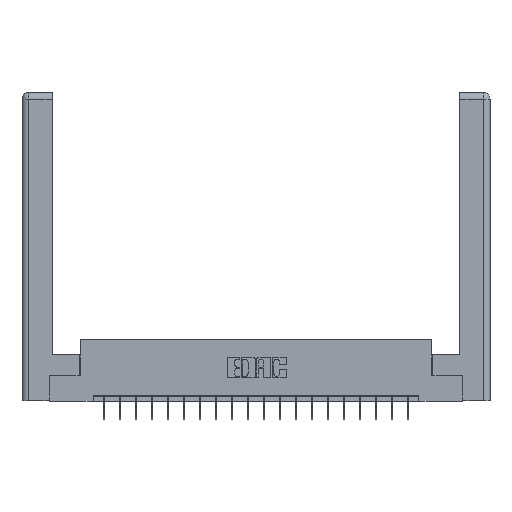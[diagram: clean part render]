
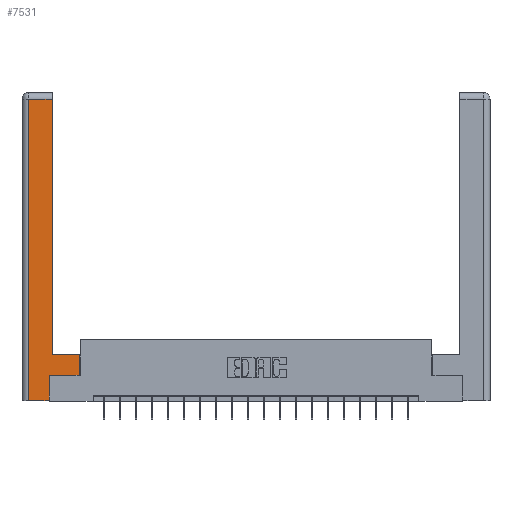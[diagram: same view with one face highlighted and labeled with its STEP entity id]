
A CAD part, top view. The second image highlights one B-rep face of the part: STEP entity #7531.
In plain terms, the highlighted planar face has unit normal (0, 0, 1).
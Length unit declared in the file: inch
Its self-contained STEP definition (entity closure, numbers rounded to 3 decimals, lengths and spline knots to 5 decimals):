
#225 = CARTESIAN_POINT ( 'NONE',  ( 0.265, 0.245, 0. ) ) ;
#317 = CARTESIAN_POINT ( 'NONE',  ( 0.0615, 0., 0. ) ) ;
#633 = DIRECTION ( 'NONE',  ( 1., 0., 0. ) ) ;
#900 = ORIENTED_EDGE ( 'NONE', *, *, #13236, .T. ) ;
#982 = CARTESIAN_POINT ( 'NONE',  ( 0.0615, 0., 0. ) ) ;
#1739 = VECTOR ( 'NONE', #633, 39.37008 ) ;
#1836 = VERTEX_POINT ( 'NONE', #8463 ) ;
#1854 = EDGE_CURVE ( 'NONE', #6002, #17932, #10151, .T. ) ;
#2524 = LINE ( 'NONE', #225, #17028 ) ;
#2531 = CARTESIAN_POINT ( 'NONE',  ( 0.0615, 2.94, 0. ) ) ;
#2778 = ORIENTED_EDGE ( 'NONE', *, *, #16266, .T. ) ;
#3439 = DIRECTION ( 'NONE',  ( 0., 0., -1. ) ) ;
#3519 = VERTEX_POINT ( 'NONE', #13654 ) ;
#3767 = CARTESIAN_POINT ( 'NONE',  ( 0.565, 0.45, 0. ) ) ;
#4159 = DIRECTION ( 'NONE',  ( -1., 0., 0. ) ) ;
#4185 = DIRECTION ( 'NONE',  ( 0., -1., 0. ) ) ;
#5205 = CARTESIAN_POINT ( 'NONE',  ( 0., 0., 0. ) ) ;
#5791 = CARTESIAN_POINT ( 'NONE',  ( 0.0615, 2.94, 0. ) ) ;
#5949 = ORIENTED_EDGE ( 'NONE', *, *, #10541, .T. ) ;
#5978 = AXIS2_PLACEMENT_3D ( 'NONE', #5205, #3439, #8343 ) ;
#6002 = VERTEX_POINT ( 'NONE', #16524 ) ;
#6455 = LINE ( 'NONE', #2531, #10020 ) ;
#7178 = VERTEX_POINT ( 'NONE', #7567 ) ;
#7236 = LINE ( 'NONE', #982, #13884 ) ;
#7531 = ADVANCED_FACE ( 'NONE', ( #19474 ), #18111, .F. ) ;
#7567 = CARTESIAN_POINT ( 'NONE',  ( 0.295, 2.94, 0. ) ) ;
#8107 = VERTEX_POINT ( 'NONE', #18086 ) ;
#8117 = LINE ( 'NONE', #13614, #1739 ) ;
#8343 = DIRECTION ( 'NONE',  ( -1., 0., 0. ) ) ;
#8373 = EDGE_LOOP ( 'NONE', ( #9507, #20205, #2778, #11912, #5949, #18914, #19604, #900 ) ) ;
#8411 = EDGE_CURVE ( 'NONE', #3519, #7178, #18422, .T. ) ;
#8463 = CARTESIAN_POINT ( 'NONE',  ( 0.265, 0.245, 0. ) ) ;
#8599 = CARTESIAN_POINT ( 'NONE',  ( 0.565, 0.45, 0. ) ) ;
#8881 = VECTOR ( 'NONE', #12105, 39.37008 ) ;
#9274 = LINE ( 'NONE', #15005, #18453 ) ;
#9507 = ORIENTED_EDGE ( 'NONE', *, *, #8411, .T. ) ;
#9956 = VERTEX_POINT ( 'NONE', #317 ) ;
#10020 = VECTOR ( 'NONE', #4159, 39.37008 ) ;
#10151 = LINE ( 'NONE', #3767, #8881 ) ;
#10386 = DIRECTION ( 'NONE',  ( 0., 1., 0. ) ) ;
#10541 = EDGE_CURVE ( 'NONE', #8107, #1836, #2524, .T. ) ;
#11912 = ORIENTED_EDGE ( 'NONE', *, *, #16694, .T. ) ;
#11979 = DIRECTION ( 'NONE',  ( -1., 0., 0. ) ) ;
#12105 = DIRECTION ( 'NONE',  ( 0., 1., 0. ) ) ;
#12991 = DIRECTION ( 'NONE',  ( 0., 1., 0. ) ) ;
#13236 = EDGE_CURVE ( 'NONE', #17932, #3519, #13496, .T. ) ;
#13265 = EDGE_CURVE ( 'NONE', #1836, #6002, #8117, .T. ) ;
#13496 = LINE ( 'NONE', #18169, #18574 ) ;
#13614 = CARTESIAN_POINT ( 'NONE',  ( 0.565, 0.245, 0. ) ) ;
#13654 = CARTESIAN_POINT ( 'NONE',  ( 0.295, 0.45, 0. ) ) ;
#13838 = VECTOR ( 'NONE', #10386, 39.37008 ) ;
#13884 = VECTOR ( 'NONE', #4185, 39.37008 ) ;
#15005 = CARTESIAN_POINT ( 'NONE',  ( 0.265, 0., 0. ) ) ;
#15440 = CARTESIAN_POINT ( 'NONE',  ( 0.295, 3., 0. ) ) ;
#16266 = EDGE_CURVE ( 'NONE', #16832, #9956, #7236, .T. ) ;
#16524 = CARTESIAN_POINT ( 'NONE',  ( 0.565, 0.245, 0. ) ) ;
#16619 = DIRECTION ( 'NONE',  ( 1., 0., 0. ) ) ;
#16694 = EDGE_CURVE ( 'NONE', #9956, #8107, #9274, .T. ) ;
#16813 = EDGE_CURVE ( 'NONE', #7178, #16832, #6455, .T. ) ;
#16832 = VERTEX_POINT ( 'NONE', #5791 ) ;
#17028 = VECTOR ( 'NONE', #12991, 39.37008 ) ;
#17932 = VERTEX_POINT ( 'NONE', #8599 ) ;
#18086 = CARTESIAN_POINT ( 'NONE',  ( 0.265, 0., 0. ) ) ;
#18111 = PLANE ( 'NONE',  #5978 ) ;
#18169 = CARTESIAN_POINT ( 'NONE',  ( 0.295, 0.45, 0. ) ) ;
#18422 = LINE ( 'NONE', #15440, #13838 ) ;
#18453 = VECTOR ( 'NONE', #16619, 39.37008 ) ;
#18574 = VECTOR ( 'NONE', #11979, 39.37008 ) ;
#18914 = ORIENTED_EDGE ( 'NONE', *, *, #13265, .T. ) ;
#19474 = FACE_OUTER_BOUND ( 'NONE', #8373, .T. ) ;
#19604 = ORIENTED_EDGE ( 'NONE', *, *, #1854, .T. ) ;
#20205 = ORIENTED_EDGE ( 'NONE', *, *, #16813, .T. ) ;
